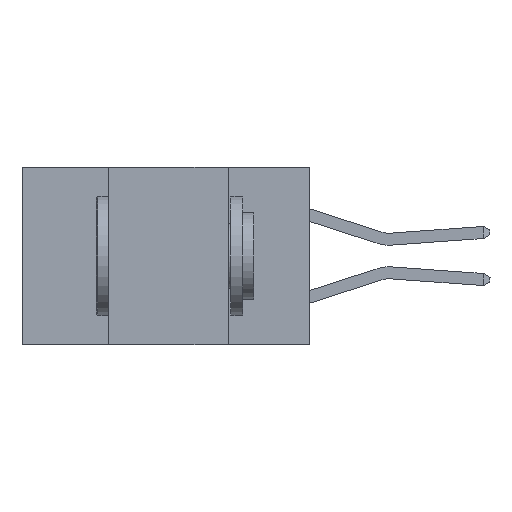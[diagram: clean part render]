
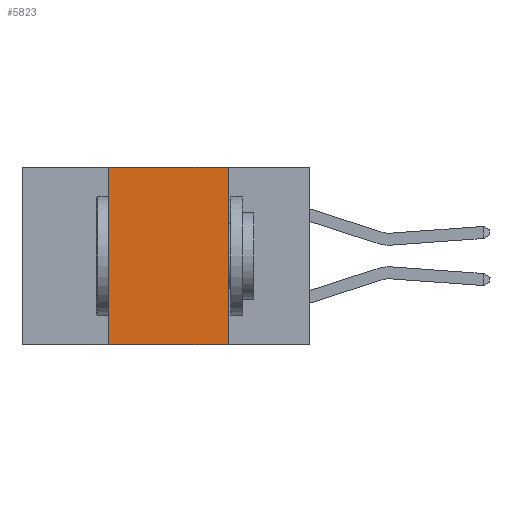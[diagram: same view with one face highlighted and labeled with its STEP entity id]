
A CAD part, left-side view. The second image highlights one B-rep face of the part: STEP entity #5823.
In plain terms, the highlighted planar face has unit normal (-1, 0, 0).
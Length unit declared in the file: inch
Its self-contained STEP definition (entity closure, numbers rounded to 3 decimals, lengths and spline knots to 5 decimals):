
#285 = CARTESIAN_POINT ( 'NONE',  ( 0., 0.17, 0. ) ) ;
#1867 = CARTESIAN_POINT ( 'NONE',  ( 0., 0.6, 0. ) ) ;
#2186 = EDGE_CURVE ( 'NONE', #9492, #22834, #23078, .T. ) ;
#3543 = VECTOR ( 'NONE', #7707, 39.37008 ) ;
#3750 = EDGE_LOOP ( 'NONE', ( #19132, #9319, #14575, #24934 ) ) ;
#3782 = DIRECTION ( 'NONE',  ( 0., -1., 0. ) ) ;
#4936 = EDGE_CURVE ( 'NONE', #21316, #22834, #25029, .T. ) ;
#5823 = ADVANCED_FACE ( 'NONE', ( #14624 ), #19460, .F. ) ;
#6912 = EDGE_CURVE ( 'NONE', #9492, #19040, #9703, .T. ) ;
#7467 = CARTESIAN_POINT ( 'NONE',  ( 0., 0.17, -0.37 ) ) ;
#7707 = DIRECTION ( 'NONE',  ( 0., 0., -1. ) ) ;
#9197 = CARTESIAN_POINT ( 'NONE',  ( 0., 0.42, 0. ) ) ;
#9319 = ORIENTED_EDGE ( 'NONE', *, *, #23697, .F. ) ;
#9492 = VERTEX_POINT ( 'NONE', #13379 ) ;
#9703 = LINE ( 'NONE', #21277, #10332 ) ;
#10332 = VECTOR ( 'NONE', #21379, 39.37008 ) ;
#13136 = VECTOR ( 'NONE', #3782, 39.37008 ) ;
#13379 = CARTESIAN_POINT ( 'NONE',  ( 0., 0.42, -0.37 ) ) ;
#14575 = ORIENTED_EDGE ( 'NONE', *, *, #6912, .F. ) ;
#14624 = FACE_OUTER_BOUND ( 'NONE', #3750, .T. ) ;
#17131 = DIRECTION ( 'NONE',  ( 0., 0., -1. ) ) ;
#17396 = DIRECTION ( 'NONE',  ( 1., 0., 0. ) ) ;
#17727 = CARTESIAN_POINT ( 'NONE',  ( 0., 0.6, 0. ) ) ;
#19040 = VERTEX_POINT ( 'NONE', #9197 ) ;
#19105 = DIRECTION ( 'NONE',  ( 0., -1., 0. ) ) ;
#19132 = ORIENTED_EDGE ( 'NONE', *, *, #4936, .F. ) ;
#19460 = PLANE ( 'NONE',  #22745 ) ;
#19605 = CARTESIAN_POINT ( 'NONE',  ( 0., 0.6, -0.37 ) ) ;
#21277 = CARTESIAN_POINT ( 'NONE',  ( 0., 0.42, -0.37 ) ) ;
#21316 = VERTEX_POINT ( 'NONE', #285 ) ;
#21379 = DIRECTION ( 'NONE',  ( 0., 0., 1. ) ) ;
#22476 = VECTOR ( 'NONE', #19105, 39.37008 ) ;
#22745 = AXIS2_PLACEMENT_3D ( 'NONE', #17727, #17396, #17131 ) ;
#22834 = VERTEX_POINT ( 'NONE', #24928 ) ;
#23078 = LINE ( 'NONE', #19605, #22476 ) ;
#23521 = LINE ( 'NONE', #1867, #13136 ) ;
#23697 = EDGE_CURVE ( 'NONE', #19040, #21316, #23521, .T. ) ;
#24928 = CARTESIAN_POINT ( 'NONE',  ( 0., 0.17, -0.37 ) ) ;
#24934 = ORIENTED_EDGE ( 'NONE', *, *, #2186, .T. ) ;
#25029 = LINE ( 'NONE', #7467, #3543 ) ;
